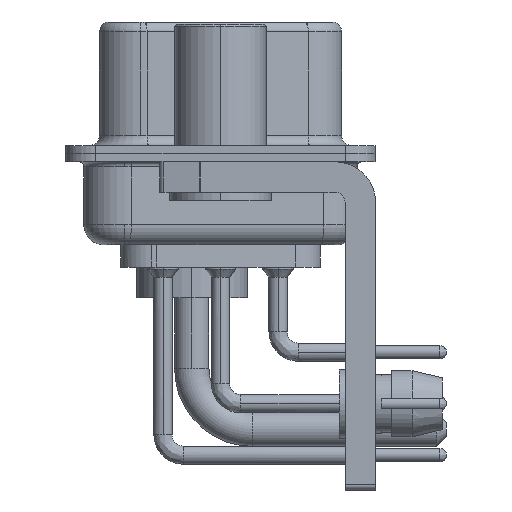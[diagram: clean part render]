
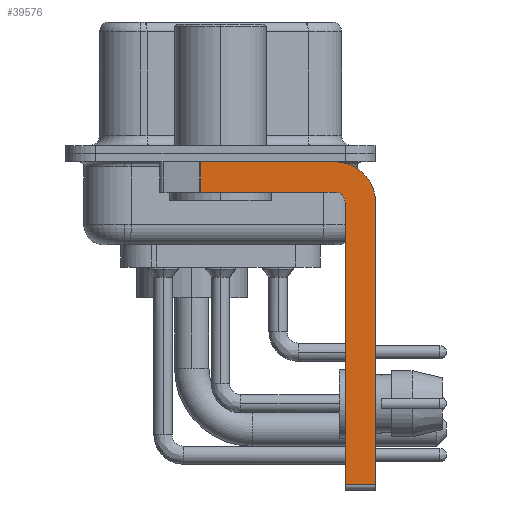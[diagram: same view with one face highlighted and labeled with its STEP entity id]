
A CAD part, left-side view. The second image highlights one B-rep face of the part: STEP entity #39576.
In plain terms, the highlighted planar face has unit normal (-1, 0, 0).
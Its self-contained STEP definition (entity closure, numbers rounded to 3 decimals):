
#909 = DIRECTION ( 'NONE',  ( 0., -1., 0. ) ) ;
#1109 = CARTESIAN_POINT ( 'NONE',  ( -2.9, -5.65, -2.4 ) ) ;
#1204 = EDGE_CURVE ( 'NONE', #7961, #33176, #17413, .T. ) ;
#1701 = EDGE_CURVE ( 'NONE', #39923, #9115, #22138, .T. ) ;
#1705 = DIRECTION ( 'NONE',  ( 0., 0., 1. ) ) ;
#2519 = EDGE_CURVE ( 'NONE', #33748, #39923, #11384, .T. ) ;
#2662 = VECTOR ( 'NONE', #9223, 1000. ) ;
#3244 = ORIENTED_EDGE ( 'NONE', *, *, #25598, .F. ) ;
#3430 = CARTESIAN_POINT ( 'NONE',  ( -2.9, -5.65, -2.4 ) ) ;
#5995 = DIRECTION ( 'NONE',  ( 0., 0., -1. ) ) ;
#6360 = ORIENTED_EDGE ( 'NONE', *, *, #1701, .F. ) ;
#7961 = VERTEX_POINT ( 'NONE', #28223 ) ;
#8108 = DIRECTION ( 'NONE',  ( -1., 0., 0. ) ) ;
#8808 = VECTOR ( 'NONE', #5995, 1000. ) ;
#9115 = VERTEX_POINT ( 'NONE', #36256 ) ;
#9124 = LINE ( 'NONE', #34754, #8808 ) ;
#9223 = DIRECTION ( 'NONE',  ( 0., 1., 0. ) ) ;
#9439 = CARTESIAN_POINT ( 'NONE',  ( -2.9, 0.978, -1.9 ) ) ;
#9575 = ORIENTED_EDGE ( 'NONE', *, *, #21356, .T. ) ;
#10116 = VECTOR ( 'NONE', #1705, 1000. ) ;
#11384 = LINE ( 'NONE', #17879, #10116 ) ;
#12637 = VERTEX_POINT ( 'NONE', #40393 ) ;
#13282 = LINE ( 'NONE', #38495, #26849 ) ;
#13517 = PLANE ( 'NONE',  #30108 ) ;
#13930 = DIRECTION ( 'NONE',  ( 0., 0., -1. ) ) ;
#15242 = VECTOR ( 'NONE', #909, 1000. ) ;
#15990 = EDGE_LOOP ( 'NONE', ( #3244, #9575, #23494, #6360, #23365, #35646, #18216, #17349 ) ) ;
#16874 = DIRECTION ( 'NONE',  ( 1., 0., 0. ) ) ;
#17045 = DIRECTION ( 'NONE',  ( 0., -1., 0. ) ) ;
#17134 = EDGE_CURVE ( 'NONE', #33748, #26973, #41264, .T. ) ;
#17349 = ORIENTED_EDGE ( 'NONE', *, *, #1204, .F. ) ;
#17413 = CIRCLE ( 'NONE', #34846, 2. ) ;
#17879 = CARTESIAN_POINT ( 'NONE',  ( -2.9, -6.15, -16.6 ) ) ;
#18216 = ORIENTED_EDGE ( 'NONE', *, *, #26392, .F. ) ;
#19106 = CARTESIAN_POINT ( 'NONE',  ( -2.9, -7.65, -2.4 ) ) ;
#19509 = LINE ( 'NONE', #32518, #2662 ) ;
#21356 = EDGE_CURVE ( 'NONE', #12637, #23433, #40980, .T. ) ;
#22138 = CIRCLE ( 'NONE', #28146, 0.5 ) ;
#22944 = CARTESIAN_POINT ( 'NONE',  ( -2.9, -5.65, -16.35 ) ) ;
#23013 = CARTESIAN_POINT ( 'NONE',  ( -2.9, 0.978, -1.9 ) ) ;
#23365 = ORIENTED_EDGE ( 'NONE', *, *, #2519, .F. ) ;
#23433 = VERTEX_POINT ( 'NONE', #23013 ) ;
#23494 = ORIENTED_EDGE ( 'NONE', *, *, #40591, .F. ) ;
#23569 = DIRECTION ( 'NONE',  ( 0., 0., -1. ) ) ;
#23590 = VECTOR ( 'NONE', #38232, 1000. ) ;
#25598 = EDGE_CURVE ( 'NONE', #12637, #7961, #13282, .T. ) ;
#26285 = DIRECTION ( 'NONE',  ( 1., 0., 0. ) ) ;
#26392 = EDGE_CURVE ( 'NONE', #33176, #26973, #9124, .T. ) ;
#26849 = VECTOR ( 'NONE', #17045, 1000. ) ;
#26973 = VERTEX_POINT ( 'NONE', #29281 ) ;
#27808 = DIRECTION ( 'NONE',  ( 0., 0., 1. ) ) ;
#28146 = AXIS2_PLACEMENT_3D ( 'NONE', #37719, #8108, #27808 ) ;
#28223 = CARTESIAN_POINT ( 'NONE',  ( -2.9, -5.65, -0.4 ) ) ;
#29281 = CARTESIAN_POINT ( 'NONE',  ( -2.9, -7.65, -16.35 ) ) ;
#30108 = AXIS2_PLACEMENT_3D ( 'NONE', #3430, #16874, #13930 ) ;
#32518 = CARTESIAN_POINT ( 'NONE',  ( -2.9, -5.65, -1.9 ) ) ;
#33176 = VERTEX_POINT ( 'NONE', #19106 ) ;
#33652 = CARTESIAN_POINT ( 'NONE',  ( -2.9, -6.15, -2.4 ) ) ;
#33748 = VERTEX_POINT ( 'NONE', #36213 ) ;
#34754 = CARTESIAN_POINT ( 'NONE',  ( -2.9, -7.65, -2.4 ) ) ;
#34846 = AXIS2_PLACEMENT_3D ( 'NONE', #1109, #26285, #23569 ) ;
#35646 = ORIENTED_EDGE ( 'NONE', *, *, #17134, .T. ) ;
#36213 = CARTESIAN_POINT ( 'NONE',  ( -2.9, -6.15, -16.35 ) ) ;
#36256 = CARTESIAN_POINT ( 'NONE',  ( -2.9, -5.65, -1.9 ) ) ;
#37719 = CARTESIAN_POINT ( 'NONE',  ( -2.9, -5.65, -2.4 ) ) ;
#38232 = DIRECTION ( 'NONE',  ( 0., 0., -1. ) ) ;
#38495 = CARTESIAN_POINT ( 'NONE',  ( -2.9, 3., -0.4 ) ) ;
#39359 = FACE_OUTER_BOUND ( 'NONE', #15990, .T. ) ;
#39576 = ADVANCED_FACE ( 'NONE', ( #39359 ), #13517, .F. ) ;
#39923 = VERTEX_POINT ( 'NONE', #33652 ) ;
#40393 = CARTESIAN_POINT ( 'NONE',  ( -2.9, 0.978, -0.4 ) ) ;
#40591 = EDGE_CURVE ( 'NONE', #9115, #23433, #19509, .T. ) ;
#40980 = LINE ( 'NONE', #9439, #23590 ) ;
#41264 = LINE ( 'NONE', #22944, #15242 ) ;
